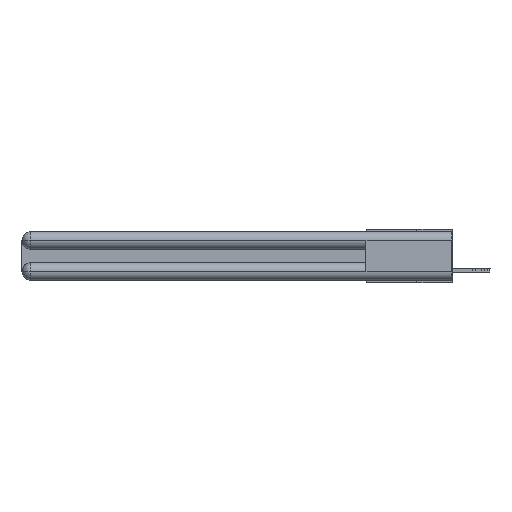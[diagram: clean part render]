
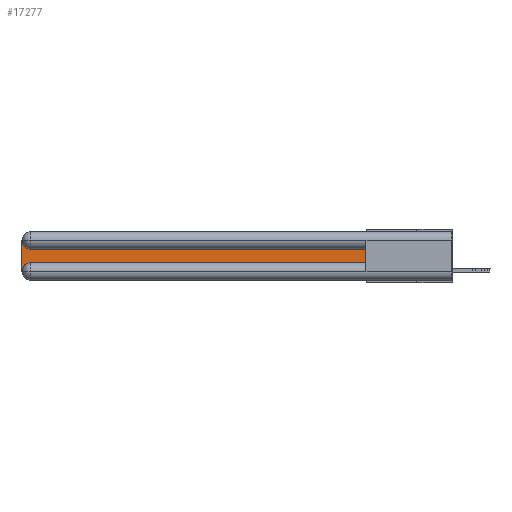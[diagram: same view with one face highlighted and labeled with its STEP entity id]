
A CAD part, left-side view. The second image highlights one B-rep face of the part: STEP entity #17277.
In plain terms, the highlighted planar face has unit normal (-1, 0, 0).
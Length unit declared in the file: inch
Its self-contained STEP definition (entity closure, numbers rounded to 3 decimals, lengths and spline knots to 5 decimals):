
#817 = DIRECTION ( 'NONE',  ( 1., 0., 0. ) ) ;
#1047 = VERTEX_POINT ( 'NONE', #2541 ) ;
#1330 = EDGE_LOOP ( 'NONE', ( #5016, #24553, #21078, #31491, #19466, #31568 ) ) ;
#2541 = CARTESIAN_POINT ( 'NONE',  ( 0.075, 0.6, -0.2175 ) ) ;
#3133 = CARTESIAN_POINT ( 'NONE',  ( 0.075, 3., -0.1225 ) ) ;
#3142 = CARTESIAN_POINT ( 'NONE',  ( 0.075, 0.6, -0.2175 ) ) ;
#3338 = CARTESIAN_POINT ( 'NONE',  ( 0.075, 2.94, -0.1225 ) ) ;
#3867 = CARTESIAN_POINT ( 'NONE',  ( 0.075, 3., -0.2175 ) ) ;
#5016 = ORIENTED_EDGE ( 'NONE', *, *, #24694, .T. ) ;
#5308 = AXIS2_PLACEMENT_3D ( 'NONE', #29224, #817, #18981 ) ;
#6088 = AXIS2_PLACEMENT_3D ( 'NONE', #26877, #19370, #32154 ) ;
#6911 = LINE ( 'NONE', #8826, #13059 ) ;
#8826 = CARTESIAN_POINT ( 'NONE',  ( 0.075, 0.6, -0.2175 ) ) ;
#9827 = CARTESIAN_POINT ( 'NONE',  ( 0.075, 0.6, -0.1225 ) ) ;
#10217 = VECTOR ( 'NONE', #12359, 39.37008 ) ;
#10654 = CARTESIAN_POINT ( 'NONE',  ( 0.075, 0.6, -0.1225 ) ) ;
#10885 = VERTEX_POINT ( 'NONE', #10654 ) ;
#11945 = VERTEX_POINT ( 'NONE', #31754 ) ;
#12359 = DIRECTION ( 'NONE',  ( 0., 1., 0. ) ) ;
#12635 = LINE ( 'NONE', #3142, #31798 ) ;
#13059 = VECTOR ( 'NONE', #17483, 39.37008 ) ;
#13314 = DIRECTION ( 'NONE',  ( 0., 0., -1. ) ) ;
#15510 = VECTOR ( 'NONE', #32519, 39.37008 ) ;
#16704 = CIRCLE ( 'NONE', #5308, 0.06 ) ;
#16803 = EDGE_CURVE ( 'NONE', #31190, #29131, #23287, .T. ) ;
#17277 = ADVANCED_FACE ( 'NONE', ( #26919 ), #29261, .F. ) ;
#17483 = DIRECTION ( 'NONE',  ( 0., 0., 1. ) ) ;
#17532 = LINE ( 'NONE', #9827, #10217 ) ;
#18005 = EDGE_CURVE ( 'NONE', #22287, #1047, #12635, .T. ) ;
#18981 = DIRECTION ( 'NONE',  ( 0., 0., -1. ) ) ;
#19370 = DIRECTION ( 'NONE',  ( 1., 0., 0. ) ) ;
#19466 = ORIENTED_EDGE ( 'NONE', *, *, #18005, .T. ) ;
#21078 = ORIENTED_EDGE ( 'NONE', *, *, #24468, .T. ) ;
#21394 = DIRECTION ( 'NONE',  ( 0., -1., 0. ) ) ;
#22287 = VERTEX_POINT ( 'NONE', #24090 ) ;
#23287 = CIRCLE ( 'NONE', #6088, 0.06 ) ;
#24090 = CARTESIAN_POINT ( 'NONE',  ( 0.075, 2.94, -0.2175 ) ) ;
#24468 = EDGE_CURVE ( 'NONE', #29131, #11945, #32663, .T. ) ;
#24553 = ORIENTED_EDGE ( 'NONE', *, *, #16803, .T. ) ;
#24694 = EDGE_CURVE ( 'NONE', #10885, #31190, #17532, .T. ) ;
#26877 = CARTESIAN_POINT ( 'NONE',  ( 0.075, 2.94, -0.0625 ) ) ;
#26919 = FACE_OUTER_BOUND ( 'NONE', #1330, .T. ) ;
#27911 = CARTESIAN_POINT ( 'NONE',  ( 0.075, 3., -0.0625 ) ) ;
#28343 = EDGE_CURVE ( 'NONE', #11945, #22287, #16704, .T. ) ;
#28443 = EDGE_CURVE ( 'NONE', #1047, #10885, #6911, .T. ) ;
#29131 = VERTEX_POINT ( 'NONE', #27911 ) ;
#29224 = CARTESIAN_POINT ( 'NONE',  ( 0.075, 2.94, -0.2775 ) ) ;
#29261 = PLANE ( 'NONE',  #32337 ) ;
#31190 = VERTEX_POINT ( 'NONE', #3338 ) ;
#31491 = ORIENTED_EDGE ( 'NONE', *, *, #28343, .T. ) ;
#31568 = ORIENTED_EDGE ( 'NONE', *, *, #28443, .T. ) ;
#31661 = DIRECTION ( 'NONE',  ( 1., 0., 0. ) ) ;
#31754 = CARTESIAN_POINT ( 'NONE',  ( 0.075, 3., -0.2775 ) ) ;
#31798 = VECTOR ( 'NONE', #21394, 39.37008 ) ;
#32154 = DIRECTION ( 'NONE',  ( 0., 0., -1. ) ) ;
#32337 = AXIS2_PLACEMENT_3D ( 'NONE', #3133, #31661, #13314 ) ;
#32519 = DIRECTION ( 'NONE',  ( 0., 0., -1. ) ) ;
#32663 = LINE ( 'NONE', #3867, #15510 ) ;
